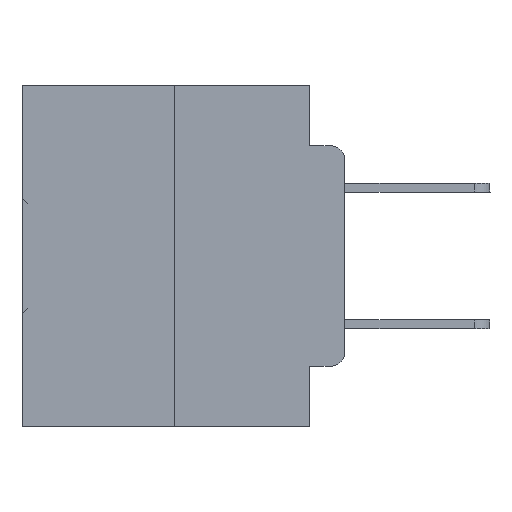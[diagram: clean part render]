
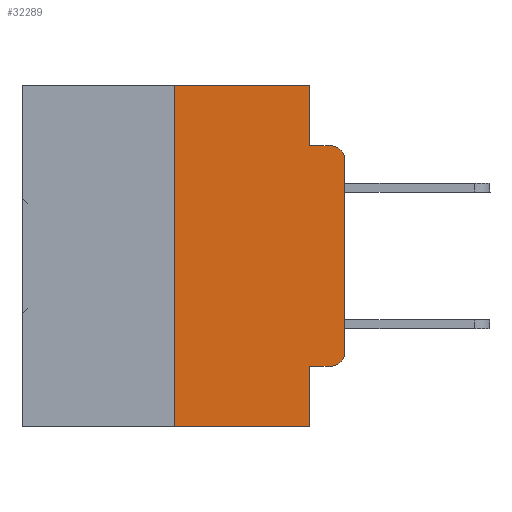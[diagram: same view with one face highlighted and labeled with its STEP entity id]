
A CAD part, left-side view. The second image highlights one B-rep face of the part: STEP entity #32289.
In plain terms, the highlighted planar face has unit normal (-1, 0, 0).
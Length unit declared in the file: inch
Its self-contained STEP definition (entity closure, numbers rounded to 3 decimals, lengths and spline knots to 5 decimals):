
#177 = DIRECTION ( 'NONE',  ( 0., -1., 0. ) ) ;
#422 = ORIENTED_EDGE ( 'NONE', *, *, #27798, .T. ) ;
#505 = CARTESIAN_POINT ( 'NONE',  ( 0., 0.051, -0.4115 ) ) ;
#620 = CARTESIAN_POINT ( 'NONE',  ( 0., 0., -0.3915 ) ) ;
#627 = DIRECTION ( 'NONE',  ( 0., 0., -1. ) ) ;
#1256 = VECTOR ( 'NONE', #28718, 39.37008 ) ;
#1331 = EDGE_CURVE ( 'NONE', #29982, #23614, #24523, .T. ) ;
#1334 = CARTESIAN_POINT ( 'NONE',  ( 0., 0.02, -0.0885 ) ) ;
#1614 = CARTESIAN_POINT ( 'NONE',  ( 0., 0.051, -0.0885 ) ) ;
#2203 = LINE ( 'NONE', #25905, #1256 ) ;
#2234 = DIRECTION ( 'NONE',  ( 0., -1., 0. ) ) ;
#3095 = PLANE ( 'NONE',  #31776 ) ;
#3233 = VECTOR ( 'NONE', #19966, 39.37008 ) ;
#3241 = DIRECTION ( 'NONE',  ( 0., 0., 1. ) ) ;
#4929 = LINE ( 'NONE', #17021, #25981 ) ;
#5193 = VERTEX_POINT ( 'NONE', #7213 ) ;
#5514 = EDGE_LOOP ( 'NONE', ( #31219, #15358, #12939, #27427, #25022, #28599, #422, #12477, #18384, #25537 ) ) ;
#5958 = FACE_OUTER_BOUND ( 'NONE', #5514, .T. ) ;
#6923 = DIRECTION ( 'NONE',  ( 0., 0., -1. ) ) ;
#7213 = CARTESIAN_POINT ( 'NONE',  ( 0., 0.25, -0.5 ) ) ;
#8273 = VECTOR ( 'NONE', #9258, 39.37008 ) ;
#8805 = DIRECTION ( 'NONE',  ( 1., 0., 0. ) ) ;
#9007 = EDGE_CURVE ( 'NONE', #22439, #29982, #4929, .T. ) ;
#9025 = VECTOR ( 'NONE', #26616, 39.37008 ) ;
#9149 = LINE ( 'NONE', #22807, #8273 ) ;
#9175 = CARTESIAN_POINT ( 'NONE',  ( 0., 0.051, -0.4115 ) ) ;
#9258 = DIRECTION ( 'NONE',  ( 0., 0., -1. ) ) ;
#9704 = EDGE_CURVE ( 'NONE', #18288, #22439, #12735, .T. ) ;
#11532 = EDGE_CURVE ( 'NONE', #13744, #18288, #25206, .T. ) ;
#12477 = ORIENTED_EDGE ( 'NONE', *, *, #16968, .F. ) ;
#12677 = AXIS2_PLACEMENT_3D ( 'NONE', #19095, #19340, #6923 ) ;
#12735 = CIRCLE ( 'NONE', #34123, 0.02 ) ;
#12939 = ORIENTED_EDGE ( 'NONE', *, *, #29847, .F. ) ;
#13225 = VERTEX_POINT ( 'NONE', #20617 ) ;
#13744 = VERTEX_POINT ( 'NONE', #9175 ) ;
#14180 = CARTESIAN_POINT ( 'NONE',  ( 0., 0.473, 0. ) ) ;
#14215 = DIRECTION ( 'NONE',  ( 0., -1., 0. ) ) ;
#14780 = CARTESIAN_POINT ( 'NONE',  ( 0., 0., -0.1085 ) ) ;
#15273 = CARTESIAN_POINT ( 'NONE',  ( 0., 0.051, 0. ) ) ;
#15358 = ORIENTED_EDGE ( 'NONE', *, *, #1331, .T. ) ;
#15542 = CARTESIAN_POINT ( 'NONE',  ( 0., 0.02, -0.4115 ) ) ;
#16968 = EDGE_CURVE ( 'NONE', #13744, #33991, #22636, .T. ) ;
#17021 = CARTESIAN_POINT ( 'NONE',  ( 0., 0., 0. ) ) ;
#17319 = DIRECTION ( 'NONE',  ( -1., 0., 0. ) ) ;
#18288 = VERTEX_POINT ( 'NONE', #15542 ) ;
#18384 = ORIENTED_EDGE ( 'NONE', *, *, #11532, .T. ) ;
#18799 = EDGE_CURVE ( 'NONE', #5193, #13225, #2203, .T. ) ;
#18831 = CARTESIAN_POINT ( 'NONE',  ( 0., 0.473, 0. ) ) ;
#19095 = CARTESIAN_POINT ( 'NONE',  ( 0., 0.02, -0.1085 ) ) ;
#19340 = DIRECTION ( 'NONE',  ( -1., 0., 0. ) ) ;
#19467 = VECTOR ( 'NONE', #2234, 39.37008 ) ;
#19966 = DIRECTION ( 'NONE',  ( 0., -1., 0. ) ) ;
#20617 = CARTESIAN_POINT ( 'NONE',  ( 0., 0.25, 0. ) ) ;
#20726 = LINE ( 'NONE', #33332, #26288 ) ;
#21543 = LINE ( 'NONE', #33352, #28891 ) ;
#22439 = VERTEX_POINT ( 'NONE', #620 ) ;
#22448 = EDGE_CURVE ( 'NONE', #34211, #29572, #9149, .T. ) ;
#22636 = LINE ( 'NONE', #23972, #9025 ) ;
#22807 = CARTESIAN_POINT ( 'NONE',  ( 0., 0.051, 0. ) ) ;
#23614 = VERTEX_POINT ( 'NONE', #1334 ) ;
#23972 = CARTESIAN_POINT ( 'NONE',  ( 0., 0.051, 0. ) ) ;
#24523 = CIRCLE ( 'NONE', #12677, 0.02 ) ;
#24737 = CARTESIAN_POINT ( 'NONE',  ( 0., 0.051, -0.5 ) ) ;
#25022 = ORIENTED_EDGE ( 'NONE', *, *, #27579, .F. ) ;
#25206 = LINE ( 'NONE', #505, #3233 ) ;
#25537 = ORIENTED_EDGE ( 'NONE', *, *, #9704, .T. ) ;
#25865 = LINE ( 'NONE', #18831, #19467 ) ;
#25905 = CARTESIAN_POINT ( 'NONE',  ( 0., 0.25, 0. ) ) ;
#25981 = VECTOR ( 'NONE', #3241, 39.37008 ) ;
#26288 = VECTOR ( 'NONE', #177, 39.37008 ) ;
#26616 = DIRECTION ( 'NONE',  ( 0., 0., -1. ) ) ;
#27427 = ORIENTED_EDGE ( 'NONE', *, *, #22448, .F. ) ;
#27579 = EDGE_CURVE ( 'NONE', #13225, #34211, #25865, .T. ) ;
#27798 = EDGE_CURVE ( 'NONE', #5193, #33991, #20726, .T. ) ;
#27933 = DIRECTION ( 'NONE',  ( 0., 0., -1. ) ) ;
#28599 = ORIENTED_EDGE ( 'NONE', *, *, #18799, .F. ) ;
#28718 = DIRECTION ( 'NONE',  ( 0., 0., 1. ) ) ;
#28891 = VECTOR ( 'NONE', #14215, 39.37008 ) ;
#29572 = VERTEX_POINT ( 'NONE', #1614 ) ;
#29847 = EDGE_CURVE ( 'NONE', #29572, #23614, #21543, .T. ) ;
#29982 = VERTEX_POINT ( 'NONE', #14780 ) ;
#31219 = ORIENTED_EDGE ( 'NONE', *, *, #9007, .T. ) ;
#31776 = AXIS2_PLACEMENT_3D ( 'NONE', #14180, #8805, #27933 ) ;
#32289 = ADVANCED_FACE ( 'NONE', ( #5958 ), #3095, .F. ) ;
#33332 = CARTESIAN_POINT ( 'NONE',  ( 0., 0.473, -0.5 ) ) ;
#33352 = CARTESIAN_POINT ( 'NONE',  ( 0., 0.051, -0.0885 ) ) ;
#33755 = CARTESIAN_POINT ( 'NONE',  ( 0., 0.02, -0.3915 ) ) ;
#33991 = VERTEX_POINT ( 'NONE', #24737 ) ;
#34123 = AXIS2_PLACEMENT_3D ( 'NONE', #33755, #17319, #627 ) ;
#34211 = VERTEX_POINT ( 'NONE', #15273 ) ;
